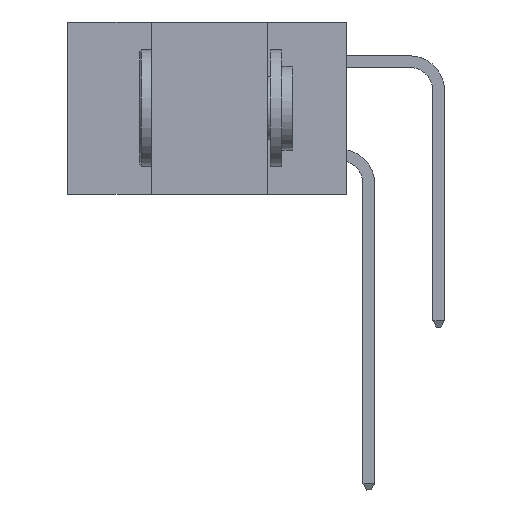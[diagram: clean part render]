
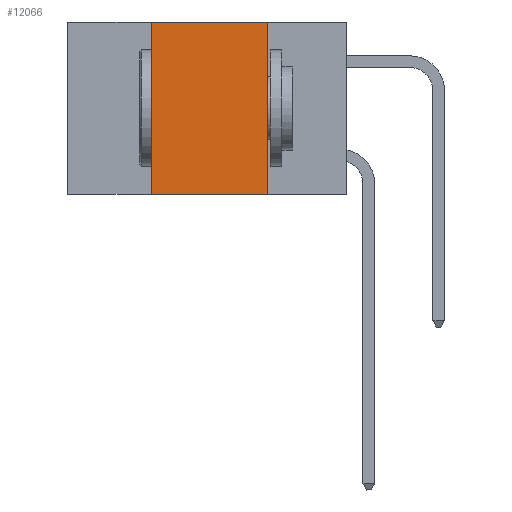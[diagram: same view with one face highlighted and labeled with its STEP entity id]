
A CAD part, left-side view. The second image highlights one B-rep face of the part: STEP entity #12066.
In plain terms, the highlighted planar face has unit normal (-1, 0, 0).
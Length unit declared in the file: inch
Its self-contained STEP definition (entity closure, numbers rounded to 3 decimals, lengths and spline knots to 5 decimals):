
#108 = ORIENTED_EDGE ( 'NONE', *, *, #4961, .F. ) ;
#466 = LINE ( 'NONE', #11794, #10373 ) ;
#600 = VECTOR ( 'NONE', #3769, 39.37008 ) ;
#923 = DIRECTION ( 'NONE',  ( 1., 0., 0. ) ) ;
#1232 = CARTESIAN_POINT ( 'NONE',  ( 0., 0.17, 0. ) ) ;
#1579 = VECTOR ( 'NONE', #3117, 39.37008 ) ;
#2137 = EDGE_LOOP ( 'NONE', ( #108, #11135, #3664, #3294 ) ) ;
#2237 = EDGE_CURVE ( 'NONE', #12865, #5746, #466, .T. ) ;
#2634 = CARTESIAN_POINT ( 'NONE',  ( 0., 0.17, 0. ) ) ;
#3117 = DIRECTION ( 'NONE',  ( 0., 0., 1. ) ) ;
#3294 = ORIENTED_EDGE ( 'NONE', *, *, #13751, .T. ) ;
#3495 = LINE ( 'NONE', #2634, #600 ) ;
#3664 = ORIENTED_EDGE ( 'NONE', *, *, #6060, .F. ) ;
#3769 = DIRECTION ( 'NONE',  ( 0., 0., -1. ) ) ;
#4150 = VECTOR ( 'NONE', #8709, 39.37008 ) ;
#4245 = AXIS2_PLACEMENT_3D ( 'NONE', #8437, #923, #9667 ) ;
#4961 = EDGE_CURVE ( 'NONE', #5746, #13098, #3495, .T. ) ;
#5746 = VERTEX_POINT ( 'NONE', #1232 ) ;
#6060 = EDGE_CURVE ( 'NONE', #15803, #12865, #11482, .T. ) ;
#6415 = FACE_OUTER_BOUND ( 'NONE', #2137, .T. ) ;
#8437 = CARTESIAN_POINT ( 'NONE',  ( 0., 0.6, 0. ) ) ;
#8709 = DIRECTION ( 'NONE',  ( 0., -1., 0. ) ) ;
#9625 = CARTESIAN_POINT ( 'NONE',  ( 0., 0.42, 0. ) ) ;
#9667 = DIRECTION ( 'NONE',  ( 0., 0., -1. ) ) ;
#10373 = VECTOR ( 'NONE', #11804, 39.37008 ) ;
#10758 = LINE ( 'NONE', #13793, #4150 ) ;
#11135 = ORIENTED_EDGE ( 'NONE', *, *, #2237, .F. ) ;
#11482 = LINE ( 'NONE', #9625, #1579 ) ;
#11794 = CARTESIAN_POINT ( 'NONE',  ( 0., 0.6, 0. ) ) ;
#11804 = DIRECTION ( 'NONE',  ( 0., -1., 0. ) ) ;
#12066 = ADVANCED_FACE ( 'NONE', ( #6415 ), #14492, .F. ) ;
#12865 = VERTEX_POINT ( 'NONE', #13126 ) ;
#13098 = VERTEX_POINT ( 'NONE', #13546 ) ;
#13126 = CARTESIAN_POINT ( 'NONE',  ( 0., 0.42, 0. ) ) ;
#13546 = CARTESIAN_POINT ( 'NONE',  ( 0., 0.17, -0.37 ) ) ;
#13751 = EDGE_CURVE ( 'NONE', #15803, #13098, #10758, .T. ) ;
#13793 = CARTESIAN_POINT ( 'NONE',  ( 0., 0.6, -0.37 ) ) ;
#14492 = PLANE ( 'NONE',  #4245 ) ;
#15314 = CARTESIAN_POINT ( 'NONE',  ( 0., 0.42, -0.37 ) ) ;
#15803 = VERTEX_POINT ( 'NONE', #15314 ) ;
